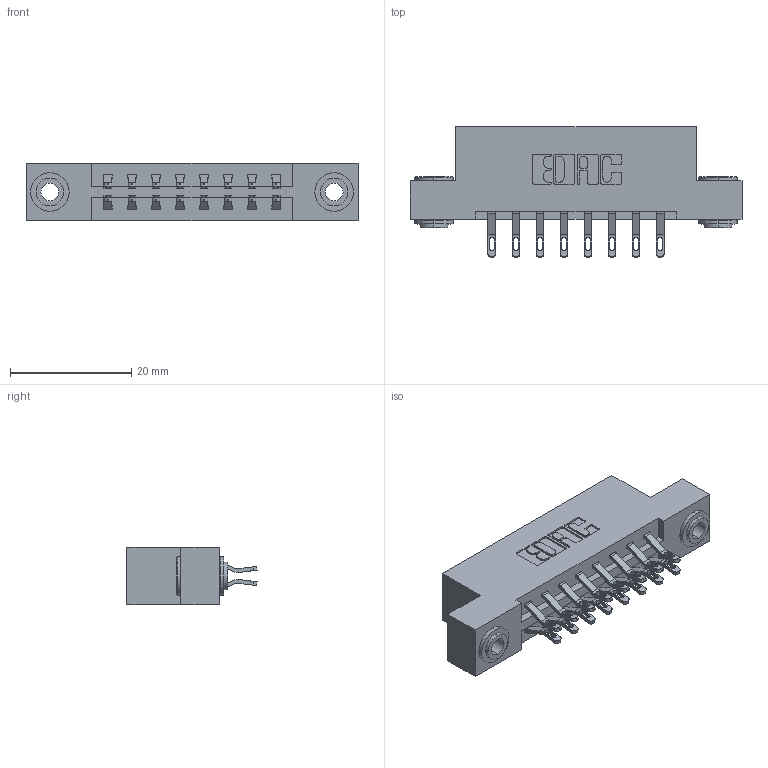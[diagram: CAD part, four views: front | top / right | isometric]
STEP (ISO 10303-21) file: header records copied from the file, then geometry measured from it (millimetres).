
FILE_DESCRIPTION (( 'STEP AP203' ), '1' );
FILE_NAME ('387-016-555-203.STEP', '2019-10-15T23:37:17', ( '' ), ( '' ), 'SwSTEP 2.0', 'SolidWorks 2016', '' );
FILE_SCHEMA (( 'CONFIG_CONTROL_DESIGN' ));
Length unit declared in the file: inch
Products named in the file (4): 337 Part_Flush Mounting Lugs - 0.156 Dia-TH; 387-016-555-203; 345-292-001_555 Tail; 345-250-002_345-250-002-102
Assembly tree (19 placements, depth 2):
  387-016-555-203
    337 Part_Flush Mounting Lugs - 0.156 Dia-TH
    345-292-001_555 Tail  x16
    345-250-002_345-250-002-102  x2
Bounding box: 54.71 x 21.47 x 9.4 mm (x, y, z)
Volume: 5379.2 mm3; surface area: 6150.2 mm2
Topology: 19 solids, 19 shells, 1112 faces, 3411 edges, 2270 vertices
Faces by surface type: plane 656, cylinder 448, cone 8
Entity records: 11576 total; most frequent: CARTESIAN_POINT 1987, ORIENTED_EDGE 1886, DIRECTION 1757, EDGE_CURVE 943, LINE 771, VECTOR 771, VERTEX_POINT 626, AXIS2_PLACEMENT_3D 493
